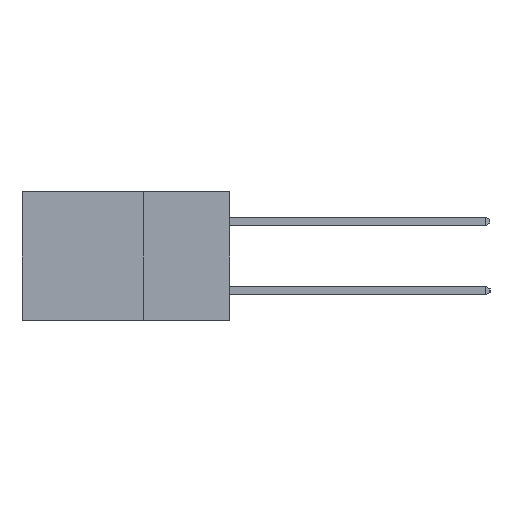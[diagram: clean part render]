
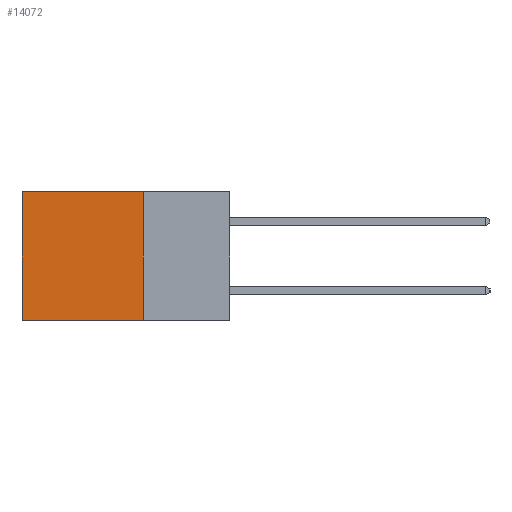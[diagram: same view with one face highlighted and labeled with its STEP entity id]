
A CAD part, left-side view. The second image highlights one B-rep face of the part: STEP entity #14072.
In plain terms, the highlighted planar face has unit normal (-1, 0, 0).
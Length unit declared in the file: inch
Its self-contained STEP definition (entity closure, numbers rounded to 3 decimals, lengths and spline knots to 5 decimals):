
#26 = EDGE_LOOP ( 'NONE', ( #9801, #12528, #11428, #379 ) ) ;
#349 = DIRECTION ( 'NONE',  ( 0., 0., -1. ) ) ;
#379 = ORIENTED_EDGE ( 'NONE', *, *, #5983, .T. ) ;
#1552 = CARTESIAN_POINT ( 'NONE',  ( 0.2615, 0.25, -0.37 ) ) ;
#2345 = LINE ( 'NONE', #8272, #8332 ) ;
#3268 = EDGE_CURVE ( 'NONE', #12363, #4024, #4975, .T. ) ;
#4024 = VERTEX_POINT ( 'NONE', #1552 ) ;
#4924 = EDGE_CURVE ( 'NONE', #11038, #6725, #12881, .T. ) ;
#4958 = DIRECTION ( 'NONE',  ( 0., 1., 0. ) ) ;
#4973 = CARTESIAN_POINT ( 'NONE',  ( 0.2615, 0.25, 0. ) ) ;
#4975 = LINE ( 'NONE', #11701, #7454 ) ;
#5845 = LINE ( 'NONE', #4973, #6247 ) ;
#5983 = EDGE_CURVE ( 'NONE', #12363, #11038, #5845, .T. ) ;
#6247 = VECTOR ( 'NONE', #4958, 39.37008 ) ;
#6725 = VERTEX_POINT ( 'NONE', #13790 ) ;
#7421 = DIRECTION ( 'NONE',  ( 1., 0., 0. ) ) ;
#7454 = VECTOR ( 'NONE', #9498, 39.37008 ) ;
#7733 = FACE_OUTER_BOUND ( 'NONE', #26, .T. ) ;
#8272 = CARTESIAN_POINT ( 'NONE',  ( 0.2615, 0.25, -0.37 ) ) ;
#8291 = CARTESIAN_POINT ( 'NONE',  ( 0.2615, 0.6, 0. ) ) ;
#8332 = VECTOR ( 'NONE', #10518, 39.37008 ) ;
#9498 = DIRECTION ( 'NONE',  ( 0., 0., -1. ) ) ;
#9615 = PLANE ( 'NONE',  #14266 ) ;
#9801 = ORIENTED_EDGE ( 'NONE', *, *, #4924, .T. ) ;
#9871 = VECTOR ( 'NONE', #14549, 39.37008 ) ;
#10518 = DIRECTION ( 'NONE',  ( 0., 1., 0. ) ) ;
#10783 = CARTESIAN_POINT ( 'NONE',  ( 0.2615, 0.25, -0.37 ) ) ;
#11038 = VERTEX_POINT ( 'NONE', #8291 ) ;
#11428 = ORIENTED_EDGE ( 'NONE', *, *, #3268, .F. ) ;
#11690 = EDGE_CURVE ( 'NONE', #4024, #6725, #2345, .T. ) ;
#11701 = CARTESIAN_POINT ( 'NONE',  ( 0.2615, 0.25, -0.37 ) ) ;
#12363 = VERTEX_POINT ( 'NONE', #14398 ) ;
#12528 = ORIENTED_EDGE ( 'NONE', *, *, #11690, .F. ) ;
#12881 = LINE ( 'NONE', #14706, #9871 ) ;
#13790 = CARTESIAN_POINT ( 'NONE',  ( 0.2615, 0.6, -0.37 ) ) ;
#14072 = ADVANCED_FACE ( 'NONE', ( #7733 ), #9615, .F. ) ;
#14266 = AXIS2_PLACEMENT_3D ( 'NONE', #10783, #7421, #349 ) ;
#14398 = CARTESIAN_POINT ( 'NONE',  ( 0.2615, 0.25, 0. ) ) ;
#14549 = DIRECTION ( 'NONE',  ( 0., 0., -1. ) ) ;
#14706 = CARTESIAN_POINT ( 'NONE',  ( 0.2615, 0.6, -0.37 ) ) ;
